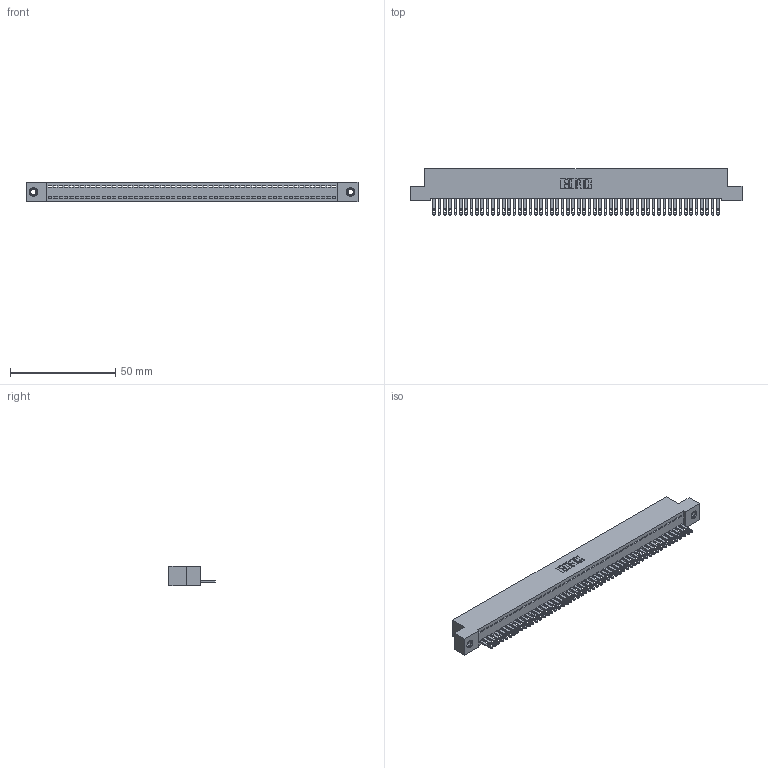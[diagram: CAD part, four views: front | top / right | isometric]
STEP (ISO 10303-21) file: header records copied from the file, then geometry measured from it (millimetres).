
FILE_DESCRIPTION (( 'STEP AP203' ), '1' );
FILE_NAME ('342-054-500-107.STEP', '2019-10-03T02:34:28', ( '' ), ( '' ), 'SwSTEP 2.0', 'SolidWorks 2016', '' );
FILE_SCHEMA (( 'CONFIG_CONTROL_DESIGN' ));
Length unit declared in the file: inch
Products named in the file (4): 342 Part_TI; 345-292-001_345-293-100; 345-250-001_345-250-005-103; 342-054-500-107
Assembly tree (57 placements, depth 2):
  342-054-500-107
    342 Part_TI
    345-292-001_345-293-100  x54
    345-250-001_345-250-005-103  x2
Bounding box: 157.48 x 21.85 x 9.4 mm (x, y, z)
Volume: 13872.8 mm3; surface area: 20734.1 mm2
Topology: 57 solids, 57 shells, 3086 faces, 9507 edges, 6330 vertices
Faces by surface type: plane 2042, cylinder 1028, cone 12, torus 4
Entity records: 32444 total; most frequent: CARTESIAN_POINT 5575, ORIENTED_EDGE 5558, DIRECTION 4713, EDGE_CURVE 2779, VECTOR 2627, LINE 2627, VERTEX_POINT 1848, AXIS2_PLACEMENT_3D 1043
